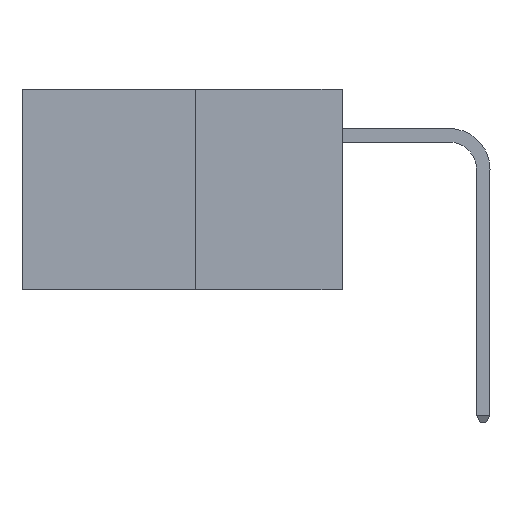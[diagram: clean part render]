
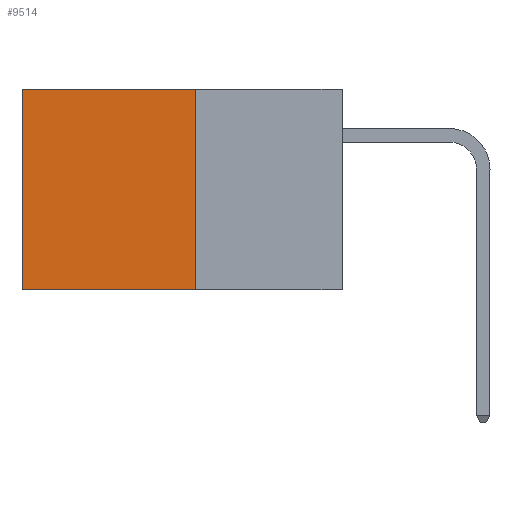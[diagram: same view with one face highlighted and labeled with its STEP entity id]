
A CAD part, left-side view. The second image highlights one B-rep face of the part: STEP entity #9514.
In plain terms, the highlighted planar face has unit normal (-1, 0, 0).
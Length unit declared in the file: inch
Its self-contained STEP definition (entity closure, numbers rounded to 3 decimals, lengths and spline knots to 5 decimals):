
#105 = FACE_OUTER_BOUND ( 'NONE', #12621, .T. ) ;
#555 = DIRECTION ( 'NONE',  ( 0., 0., -1. ) ) ;
#574 = PLANE ( 'NONE',  #7937 ) ;
#847 = CARTESIAN_POINT ( 'NONE',  ( 0.277, 0.27, -0.37 ) ) ;
#978 = ORIENTED_EDGE ( 'NONE', *, *, #9123, .T. ) ;
#3109 = LINE ( 'NONE', #12310, #15200 ) ;
#3143 = DIRECTION ( 'NONE',  ( 1., 0., 0. ) ) ;
#3432 = DIRECTION ( 'NONE',  ( 0., 0., -1. ) ) ;
#3979 = VECTOR ( 'NONE', #555, 39.37008 ) ;
#4107 = LINE ( 'NONE', #847, #8220 ) ;
#4373 = LINE ( 'NONE', #15558, #3979 ) ;
#5789 = EDGE_CURVE ( 'NONE', #14874, #15291, #4373, .T. ) ;
#6045 = ORIENTED_EDGE ( 'NONE', *, *, #7324, .F. ) ;
#6321 = ORIENTED_EDGE ( 'NONE', *, *, #5789, .T. ) ;
#6387 = CARTESIAN_POINT ( 'NONE',  ( 0.277, 0.27, -0.37 ) ) ;
#6688 = CARTESIAN_POINT ( 'NONE',  ( 0.277, 0.59, 0. ) ) ;
#7324 = EDGE_CURVE ( 'NONE', #11770, #15291, #15823, .T. ) ;
#7751 = EDGE_CURVE ( 'NONE', #11041, #11770, #4107, .T. ) ;
#7937 = AXIS2_PLACEMENT_3D ( 'NONE', #9358, #3143, #11862 ) ;
#8220 = VECTOR ( 'NONE', #3432, 39.37008 ) ;
#8655 = DIRECTION ( 'NONE',  ( 0., 1., 0. ) ) ;
#9123 = EDGE_CURVE ( 'NONE', #11041, #14874, #3109, .T. ) ;
#9358 = CARTESIAN_POINT ( 'NONE',  ( 0.277, 0.27, -0.37 ) ) ;
#9514 = ADVANCED_FACE ( 'NONE', ( #105 ), #574, .F. ) ;
#9875 = CARTESIAN_POINT ( 'NONE',  ( 0.277, 0.59, -0.37 ) ) ;
#10146 = DIRECTION ( 'NONE',  ( 0., 1., 0. ) ) ;
#10453 = CARTESIAN_POINT ( 'NONE',  ( 0.277, 0.27, -0.37 ) ) ;
#11041 = VERTEX_POINT ( 'NONE', #13502 ) ;
#11770 = VERTEX_POINT ( 'NONE', #10453 ) ;
#11862 = DIRECTION ( 'NONE',  ( 0., 0., -1. ) ) ;
#12310 = CARTESIAN_POINT ( 'NONE',  ( 0.277, 0.27, 0. ) ) ;
#12508 = VECTOR ( 'NONE', #10146, 39.37008 ) ;
#12621 = EDGE_LOOP ( 'NONE', ( #6321, #6045, #15309, #978 ) ) ;
#13502 = CARTESIAN_POINT ( 'NONE',  ( 0.277, 0.27, 0. ) ) ;
#14874 = VERTEX_POINT ( 'NONE', #6688 ) ;
#15200 = VECTOR ( 'NONE', #8655, 39.37008 ) ;
#15291 = VERTEX_POINT ( 'NONE', #9875 ) ;
#15309 = ORIENTED_EDGE ( 'NONE', *, *, #7751, .F. ) ;
#15558 = CARTESIAN_POINT ( 'NONE',  ( 0.277, 0.59, -0.37 ) ) ;
#15823 = LINE ( 'NONE', #6387, #12508 ) ;
